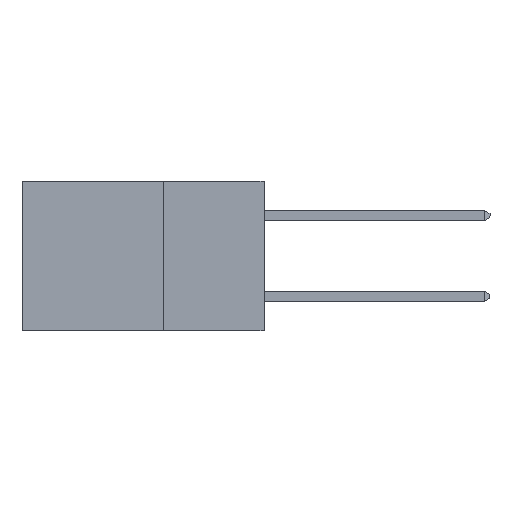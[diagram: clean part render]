
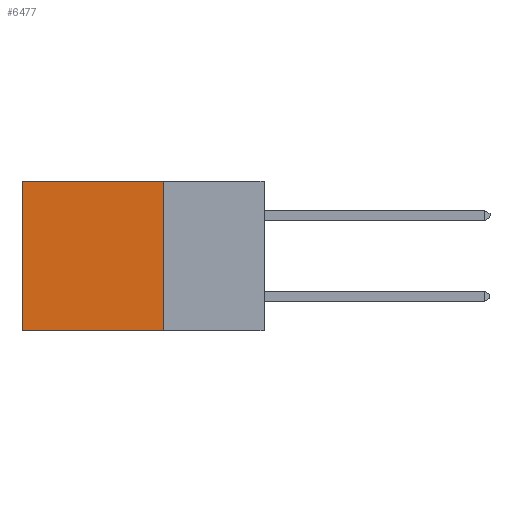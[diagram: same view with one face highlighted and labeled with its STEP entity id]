
A CAD part, left-side view. The second image highlights one B-rep face of the part: STEP entity #6477.
In plain terms, the highlighted planar face has unit normal (-1, 0, 0).
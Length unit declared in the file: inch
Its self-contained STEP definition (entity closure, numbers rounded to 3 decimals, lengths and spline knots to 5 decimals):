
#182 = CARTESIAN_POINT ( 'NONE',  ( 0.298, 0.25, 0. ) ) ;
#234 = DIRECTION ( 'NONE',  ( 0., 1., 0. ) ) ;
#637 = CARTESIAN_POINT ( 'NONE',  ( 0.298, 0.25, -0.37 ) ) ;
#1149 = EDGE_LOOP ( 'NONE', ( #14845, #16347, #6545, #9785 ) ) ;
#1941 = EDGE_CURVE ( 'NONE', #12884, #10001, #16025, .T. ) ;
#2462 = AXIS2_PLACEMENT_3D ( 'NONE', #3452, #12278, #4710 ) ;
#3452 = CARTESIAN_POINT ( 'NONE',  ( 0.298, 0.25, 0. ) ) ;
#3952 = DIRECTION ( 'NONE',  ( 0., 0., -1. ) ) ;
#4710 = DIRECTION ( 'NONE',  ( 0., 0., -1. ) ) ;
#4903 = VECTOR ( 'NONE', #11614, 39.37008 ) ;
#5314 = LINE ( 'NONE', #10378, #4903 ) ;
#5698 = VECTOR ( 'NONE', #234, 39.37008 ) ;
#6477 = ADVANCED_FACE ( 'NONE', ( #9063 ), #16064, .F. ) ;
#6545 = ORIENTED_EDGE ( 'NONE', *, *, #1941, .F. ) ;
#6936 = CARTESIAN_POINT ( 'NONE',  ( 0.298, 0.25, 0. ) ) ;
#8669 = EDGE_CURVE ( 'NONE', #12884, #11825, #15805, .T. ) ;
#8709 = EDGE_CURVE ( 'NONE', #10001, #9072, #5314, .T. ) ;
#9063 = FACE_OUTER_BOUND ( 'NONE', #1149, .T. ) ;
#9072 = VERTEX_POINT ( 'NONE', #9856 ) ;
#9785 = ORIENTED_EDGE ( 'NONE', *, *, #8669, .T. ) ;
#9856 = CARTESIAN_POINT ( 'NONE',  ( 0.298, 0.6, -0.37 ) ) ;
#10001 = VERTEX_POINT ( 'NONE', #637 ) ;
#10285 = CARTESIAN_POINT ( 'NONE',  ( 0.298, 0.6, 0. ) ) ;
#10378 = CARTESIAN_POINT ( 'NONE',  ( 0.298, 0.25, -0.37 ) ) ;
#11614 = DIRECTION ( 'NONE',  ( 0., 1., 0. ) ) ;
#11825 = VERTEX_POINT ( 'NONE', #15523 ) ;
#12278 = DIRECTION ( 'NONE',  ( 1., 0., 0. ) ) ;
#12279 = VECTOR ( 'NONE', #3952, 39.37008 ) ;
#12645 = VECTOR ( 'NONE', #15851, 39.37008 ) ;
#12689 = LINE ( 'NONE', #10285, #12279 ) ;
#12884 = VERTEX_POINT ( 'NONE', #6936 ) ;
#13336 = EDGE_CURVE ( 'NONE', #11825, #9072, #12689, .T. ) ;
#14845 = ORIENTED_EDGE ( 'NONE', *, *, #13336, .T. ) ;
#15329 = CARTESIAN_POINT ( 'NONE',  ( 0.298, 0.25, 0. ) ) ;
#15523 = CARTESIAN_POINT ( 'NONE',  ( 0.298, 0.6, 0. ) ) ;
#15805 = LINE ( 'NONE', #15329, #5698 ) ;
#15851 = DIRECTION ( 'NONE',  ( 0., 0., -1. ) ) ;
#16025 = LINE ( 'NONE', #182, #12645 ) ;
#16064 = PLANE ( 'NONE',  #2462 ) ;
#16347 = ORIENTED_EDGE ( 'NONE', *, *, #8709, .F. ) ;
